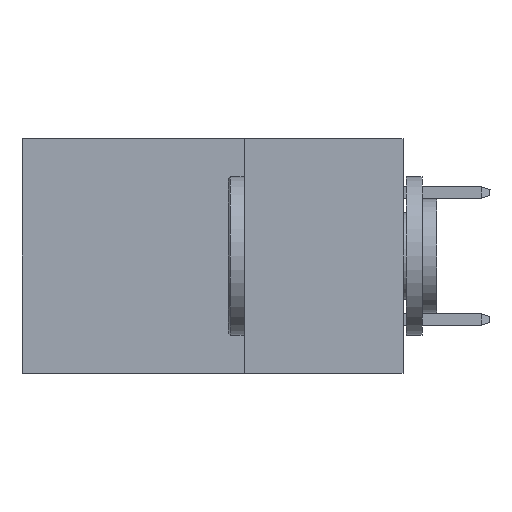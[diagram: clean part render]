
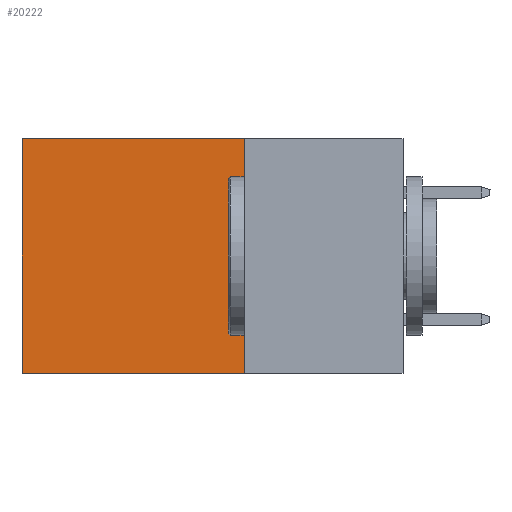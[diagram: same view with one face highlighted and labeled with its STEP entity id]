
A CAD part, left-side view. The second image highlights one B-rep face of the part: STEP entity #20222.
In plain terms, the highlighted planar face has unit normal (-1, 0, 0).
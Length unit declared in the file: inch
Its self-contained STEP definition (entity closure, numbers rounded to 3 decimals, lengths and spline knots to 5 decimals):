
#2097 = VERTEX_POINT ( 'NONE', #11245 ) ;
#6639 = EDGE_CURVE ( 'NONE', #10951, #2097, #38715, .T. ) ;
#8315 = VECTOR ( 'NONE', #30904, 39.37008 ) ;
#8682 = VECTOR ( 'NONE', #20792, 39.37008 ) ;
#10661 = EDGE_LOOP ( 'NONE', ( #12340, #43280, #20948, #32596 ) ) ;
#10951 = VERTEX_POINT ( 'NONE', #33715 ) ;
#11245 = CARTESIAN_POINT ( 'NONE',  ( 0.2875, 0.25, -0.37 ) ) ;
#12340 = ORIENTED_EDGE ( 'NONE', *, *, #21612, .T. ) ;
#12649 = PLANE ( 'NONE',  #19413 ) ;
#16023 = CARTESIAN_POINT ( 'NONE',  ( 0.2875, 0.6, -0.37 ) ) ;
#16289 = CARTESIAN_POINT ( 'NONE',  ( 0.2875, 0.25, 0. ) ) ;
#17130 = CARTESIAN_POINT ( 'NONE',  ( 0.2875, 0.25, 0. ) ) ;
#17301 = CARTESIAN_POINT ( 'NONE',  ( 0.2875, 0.6, 0. ) ) ;
#19413 = AXIS2_PLACEMENT_3D ( 'NONE', #16289, #30126, #37911 ) ;
#20049 = LINE ( 'NONE', #44663, #34281 ) ;
#20222 = ADVANCED_FACE ( 'NONE', ( #26871 ), #12649, .F. ) ;
#20792 = DIRECTION ( 'NONE',  ( 0., 0., -1. ) ) ;
#20948 = ORIENTED_EDGE ( 'NONE', *, *, #6639, .F. ) ;
#21612 = EDGE_CURVE ( 'NONE', #43318, #28809, #40993, .T. ) ;
#23004 = LINE ( 'NONE', #36369, #27114 ) ;
#26871 = FACE_OUTER_BOUND ( 'NONE', #10661, .T. ) ;
#27114 = VECTOR ( 'NONE', #29948, 39.37008 ) ;
#27164 = DIRECTION ( 'NONE',  ( 0., 1., 0. ) ) ;
#28809 = VERTEX_POINT ( 'NONE', #16023 ) ;
#29219 = EDGE_CURVE ( 'NONE', #2097, #28809, #20049, .T. ) ;
#29948 = DIRECTION ( 'NONE',  ( 0., 1., 0. ) ) ;
#30126 = DIRECTION ( 'NONE',  ( 1., 0., 0. ) ) ;
#30904 = DIRECTION ( 'NONE',  ( 0., 0., -1. ) ) ;
#32406 = EDGE_CURVE ( 'NONE', #10951, #43318, #23004, .T. ) ;
#32596 = ORIENTED_EDGE ( 'NONE', *, *, #32406, .T. ) ;
#33715 = CARTESIAN_POINT ( 'NONE',  ( 0.2875, 0.25, 0. ) ) ;
#34281 = VECTOR ( 'NONE', #27164, 39.37008 ) ;
#36369 = CARTESIAN_POINT ( 'NONE',  ( 0.2875, 0.25, 0. ) ) ;
#37911 = DIRECTION ( 'NONE',  ( 0., 0., -1. ) ) ;
#38715 = LINE ( 'NONE', #17130, #8682 ) ;
#40993 = LINE ( 'NONE', #17301, #8315 ) ;
#43280 = ORIENTED_EDGE ( 'NONE', *, *, #29219, .F. ) ;
#43318 = VERTEX_POINT ( 'NONE', #44522 ) ;
#44522 = CARTESIAN_POINT ( 'NONE',  ( 0.2875, 0.6, 0. ) ) ;
#44663 = CARTESIAN_POINT ( 'NONE',  ( 0.2875, 0.25, -0.37 ) ) ;
